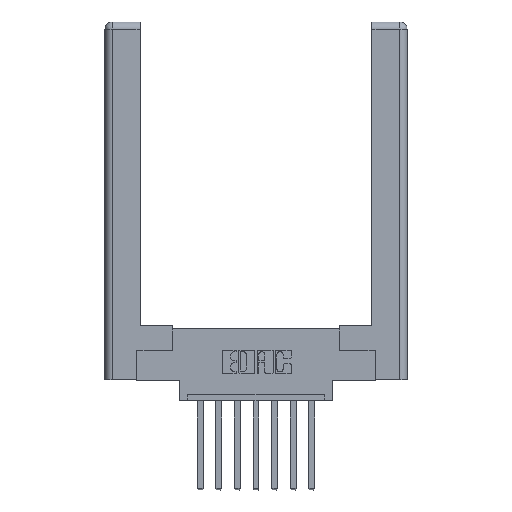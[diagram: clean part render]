
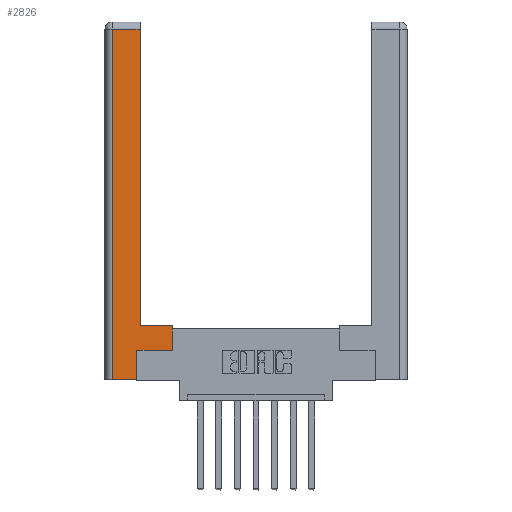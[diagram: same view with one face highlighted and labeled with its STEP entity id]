
A CAD part, top view. The second image highlights one B-rep face of the part: STEP entity #2826.
In plain terms, the highlighted planar face has unit normal (0, 0, 1).
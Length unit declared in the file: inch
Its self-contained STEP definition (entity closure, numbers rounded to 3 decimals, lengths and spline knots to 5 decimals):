
#33 = ORIENTED_EDGE ( 'NONE', *, *, #11532, .T. ) ;
#109 = LINE ( 'NONE', #413, #7237 ) ;
#128 = PLANE ( 'NONE',  #8053 ) ;
#165 = CARTESIAN_POINT ( 'NONE',  ( 0.0615, 0., 0. ) ) ;
#374 = VECTOR ( 'NONE', #7040, 39.37008 ) ;
#413 = CARTESIAN_POINT ( 'NONE',  ( 0.265, 0., 0. ) ) ;
#636 = VECTOR ( 'NONE', #12069, 39.37008 ) ;
#674 = LINE ( 'NONE', #11858, #374 ) ;
#745 = DIRECTION ( 'NONE',  ( 0., 1., 0. ) ) ;
#912 = EDGE_CURVE ( 'NONE', #7797, #5998, #8935, .T. ) ;
#1211 = DIRECTION ( 'NONE',  ( -1., 0., 0. ) ) ;
#1452 = FACE_OUTER_BOUND ( 'NONE', #4677, .T. ) ;
#2468 = ORIENTED_EDGE ( 'NONE', *, *, #4488, .T. ) ;
#2492 = ORIENTED_EDGE ( 'NONE', *, *, #9118, .T. ) ;
#2513 = VERTEX_POINT ( 'NONE', #10944 ) ;
#2530 = CARTESIAN_POINT ( 'NONE',  ( 0.565, 0.245, 0. ) ) ;
#2573 = EDGE_CURVE ( 'NONE', #8542, #2513, #7530, .T. ) ;
#2690 = DIRECTION ( 'NONE',  ( 0., 1., 0. ) ) ;
#2826 = ADVANCED_FACE ( 'NONE', ( #1452 ), #128, .F. ) ;
#3007 = CARTESIAN_POINT ( 'NONE',  ( 0.0615, 2.94, 0. ) ) ;
#3152 = LINE ( 'NONE', #2530, #636 ) ;
#3227 = EDGE_CURVE ( 'NONE', #2513, #10746, #11723, .T. ) ;
#3265 = DIRECTION ( 'NONE',  ( 1., 0., 0. ) ) ;
#3267 = EDGE_CURVE ( 'NONE', #5998, #9427, #109, .T. ) ;
#4218 = EDGE_CURVE ( 'NONE', #9445, #7797, #10954, .T. ) ;
#4488 = EDGE_CURVE ( 'NONE', #10746, #9445, #674, .T. ) ;
#4677 = EDGE_LOOP ( 'NONE', ( #2468, #10486, #8729, #11251, #2492, #33, #11932, #11130 ) ) ;
#4824 = CARTESIAN_POINT ( 'NONE',  ( 0.0615, 0., 0. ) ) ;
#5998 = VERTEX_POINT ( 'NONE', #4824 ) ;
#6861 = CARTESIAN_POINT ( 'NONE',  ( 0.265, 0.245, 0. ) ) ;
#7040 = DIRECTION ( 'NONE',  ( 0., 1., 0. ) ) ;
#7057 = DIRECTION ( 'NONE',  ( -1., 0., 0. ) ) ;
#7237 = VECTOR ( 'NONE', #3265, 39.37008 ) ;
#7530 = LINE ( 'NONE', #9327, #10095 ) ;
#7797 = VERTEX_POINT ( 'NONE', #3007 ) ;
#7813 = VECTOR ( 'NONE', #2690, 39.37008 ) ;
#7968 = VECTOR ( 'NONE', #1211, 39.37008 ) ;
#8053 = AXIS2_PLACEMENT_3D ( 'NONE', #9975, #12184, #9367 ) ;
#8536 = CARTESIAN_POINT ( 'NONE',  ( 0.565, 0.245, 0. ) ) ;
#8542 = VERTEX_POINT ( 'NONE', #8536 ) ;
#8729 = ORIENTED_EDGE ( 'NONE', *, *, #912, .T. ) ;
#8736 = CARTESIAN_POINT ( 'NONE',  ( 0.295, 2.94, 0. ) ) ;
#8935 = LINE ( 'NONE', #165, #11177 ) ;
#9118 = EDGE_CURVE ( 'NONE', #9427, #9452, #10384, .T. ) ;
#9327 = CARTESIAN_POINT ( 'NONE',  ( 0.565, 0.45, 0. ) ) ;
#9367 = DIRECTION ( 'NONE',  ( -1., 0., 0. ) ) ;
#9427 = VERTEX_POINT ( 'NONE', #10740 ) ;
#9445 = VERTEX_POINT ( 'NONE', #8736 ) ;
#9452 = VERTEX_POINT ( 'NONE', #6861 ) ;
#9535 = CARTESIAN_POINT ( 'NONE',  ( 0.295, 0.45, 0. ) ) ;
#9607 = DIRECTION ( 'NONE',  ( 0., -1., 0. ) ) ;
#9975 = CARTESIAN_POINT ( 'NONE',  ( 0., 0., 0. ) ) ;
#10028 = CARTESIAN_POINT ( 'NONE',  ( 0.295, 0.45, 0. ) ) ;
#10095 = VECTOR ( 'NONE', #745, 39.37008 ) ;
#10384 = LINE ( 'NONE', #11198, #7813 ) ;
#10486 = ORIENTED_EDGE ( 'NONE', *, *, #4218, .T. ) ;
#10740 = CARTESIAN_POINT ( 'NONE',  ( 0.265, 0., 0. ) ) ;
#10746 = VERTEX_POINT ( 'NONE', #10028 ) ;
#10760 = CARTESIAN_POINT ( 'NONE',  ( 0.0615, 2.94, 0. ) ) ;
#10944 = CARTESIAN_POINT ( 'NONE',  ( 0.565, 0.45, 0. ) ) ;
#10954 = LINE ( 'NONE', #10760, #12144 ) ;
#11130 = ORIENTED_EDGE ( 'NONE', *, *, #3227, .T. ) ;
#11177 = VECTOR ( 'NONE', #9607, 39.37008 ) ;
#11198 = CARTESIAN_POINT ( 'NONE',  ( 0.265, 0.245, 0. ) ) ;
#11251 = ORIENTED_EDGE ( 'NONE', *, *, #3267, .T. ) ;
#11532 = EDGE_CURVE ( 'NONE', #9452, #8542, #3152, .T. ) ;
#11723 = LINE ( 'NONE', #9535, #7968 ) ;
#11858 = CARTESIAN_POINT ( 'NONE',  ( 0.295, 3., 0. ) ) ;
#11932 = ORIENTED_EDGE ( 'NONE', *, *, #2573, .T. ) ;
#12069 = DIRECTION ( 'NONE',  ( 1., 0., 0. ) ) ;
#12144 = VECTOR ( 'NONE', #7057, 39.37008 ) ;
#12184 = DIRECTION ( 'NONE',  ( 0., 0., -1. ) ) ;
